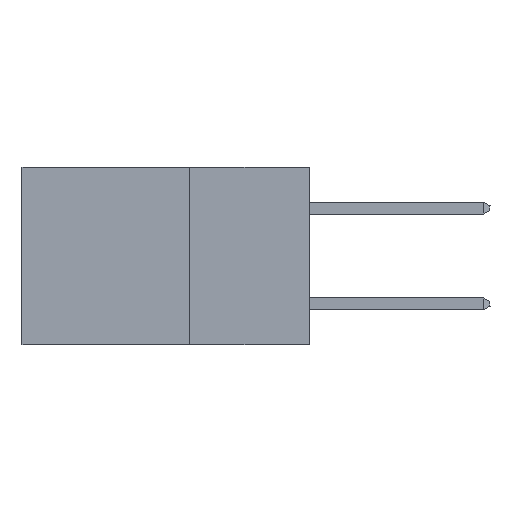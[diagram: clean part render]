
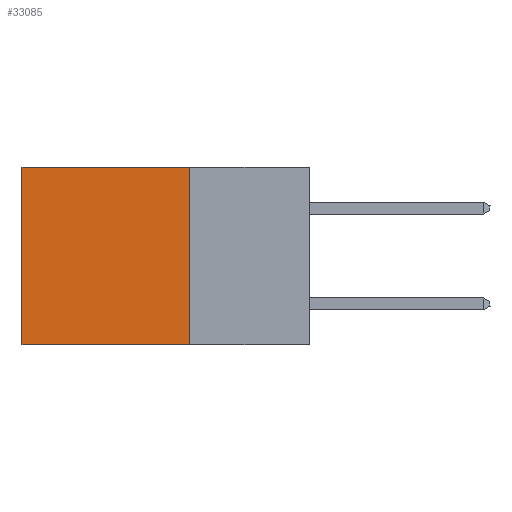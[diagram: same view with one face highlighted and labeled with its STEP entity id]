
A CAD part, left-side view. The second image highlights one B-rep face of the part: STEP entity #33085.
In plain terms, the highlighted planar face has unit normal (-1, 0, 0).
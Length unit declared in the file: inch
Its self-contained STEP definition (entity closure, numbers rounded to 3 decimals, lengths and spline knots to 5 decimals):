
#856 = EDGE_CURVE ( 'NONE', #30183, #17417, #26266, .T. ) ;
#1306 = VECTOR ( 'NONE', #34232, 39.37008 ) ;
#3551 = DIRECTION ( 'NONE',  ( 1., 0., 0. ) ) ;
#3854 = CARTESIAN_POINT ( 'NONE',  ( 0.2875, 0.25, 0. ) ) ;
#5163 = CARTESIAN_POINT ( 'NONE',  ( 0.2875, 0.6, 0. ) ) ;
#5357 = CARTESIAN_POINT ( 'NONE',  ( 0.2875, 0.6, -0.37 ) ) ;
#8350 = DIRECTION ( 'NONE',  ( 0., 1., 0. ) ) ;
#9861 = VERTEX_POINT ( 'NONE', #21894 ) ;
#10477 = AXIS2_PLACEMENT_3D ( 'NONE', #23433, #3551, #31592 ) ;
#11768 = LINE ( 'NONE', #34695, #1306 ) ;
#11921 = LINE ( 'NONE', #28826, #28114 ) ;
#13979 = CARTESIAN_POINT ( 'NONE',  ( 0.2875, 0.25, 0. ) ) ;
#14136 = EDGE_CURVE ( 'NONE', #9861, #16137, #11921, .T. ) ;
#14168 = ORIENTED_EDGE ( 'NONE', *, *, #14136, .F. ) ;
#15727 = FACE_OUTER_BOUND ( 'NONE', #19271, .T. ) ;
#16137 = VERTEX_POINT ( 'NONE', #5357 ) ;
#17417 = VERTEX_POINT ( 'NONE', #5163 ) ;
#17852 = DIRECTION ( 'NONE',  ( 0., 1., 0. ) ) ;
#19271 = EDGE_LOOP ( 'NONE', ( #20330, #14168, #29863, #33805 ) ) ;
#19500 = CARTESIAN_POINT ( 'NONE',  ( 0.2875, 0.25, 0. ) ) ;
#20330 = ORIENTED_EDGE ( 'NONE', *, *, #20405, .T. ) ;
#20405 = EDGE_CURVE ( 'NONE', #17417, #16137, #11768, .T. ) ;
#21894 = CARTESIAN_POINT ( 'NONE',  ( 0.2875, 0.25, -0.37 ) ) ;
#22797 = VECTOR ( 'NONE', #8350, 39.37008 ) ;
#23433 = CARTESIAN_POINT ( 'NONE',  ( 0.2875, 0.25, 0. ) ) ;
#25029 = LINE ( 'NONE', #3854, #26277 ) ;
#26266 = LINE ( 'NONE', #13979, #22797 ) ;
#26277 = VECTOR ( 'NONE', #34830, 39.37008 ) ;
#28114 = VECTOR ( 'NONE', #17852, 39.37008 ) ;
#28575 = PLANE ( 'NONE',  #10477 ) ;
#28826 = CARTESIAN_POINT ( 'NONE',  ( 0.2875, 0.25, -0.37 ) ) ;
#29863 = ORIENTED_EDGE ( 'NONE', *, *, #31889, .F. ) ;
#30183 = VERTEX_POINT ( 'NONE', #19500 ) ;
#31592 = DIRECTION ( 'NONE',  ( 0., 0., -1. ) ) ;
#31889 = EDGE_CURVE ( 'NONE', #30183, #9861, #25029, .T. ) ;
#33085 = ADVANCED_FACE ( 'NONE', ( #15727 ), #28575, .F. ) ;
#33805 = ORIENTED_EDGE ( 'NONE', *, *, #856, .T. ) ;
#34232 = DIRECTION ( 'NONE',  ( 0., 0., -1. ) ) ;
#34695 = CARTESIAN_POINT ( 'NONE',  ( 0.2875, 0.6, 0. ) ) ;
#34830 = DIRECTION ( 'NONE',  ( 0., 0., -1. ) ) ;
